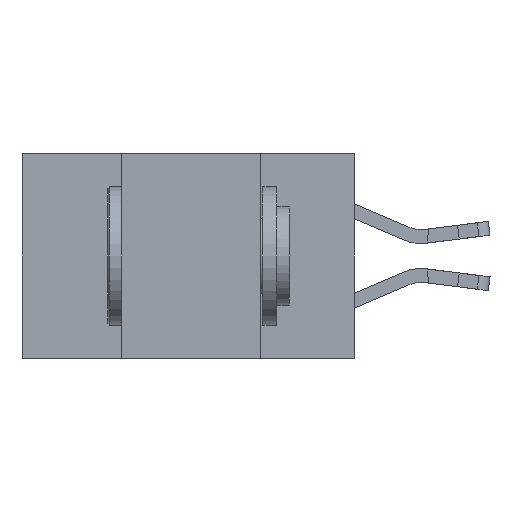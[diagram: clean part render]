
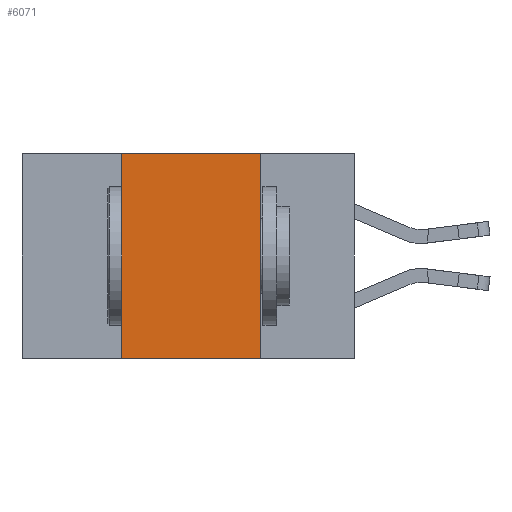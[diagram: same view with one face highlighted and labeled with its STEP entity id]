
A CAD part, left-side view. The second image highlights one B-rep face of the part: STEP entity #6071.
In plain terms, the highlighted planar face has unit normal (-1, 0, 0).
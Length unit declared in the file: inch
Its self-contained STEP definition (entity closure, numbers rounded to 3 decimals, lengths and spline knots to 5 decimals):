
#549 = DIRECTION ( 'NONE',  ( 0., -1., 0. ) ) ;
#946 = CARTESIAN_POINT ( 'NONE',  ( 0., 0.6, 0. ) ) ;
#1164 = CARTESIAN_POINT ( 'NONE',  ( 0., 0.17, 0. ) ) ;
#1494 = AXIS2_PLACEMENT_3D ( 'NONE', #2939, #2865, #2854 ) ;
#1776 = EDGE_CURVE ( 'NONE', #9136, #8596, #9429, .T. ) ;
#1821 = LINE ( 'NONE', #5766, #6699 ) ;
#2854 = DIRECTION ( 'NONE',  ( 0., 0., -1. ) ) ;
#2865 = DIRECTION ( 'NONE',  ( 1., 0., 0. ) ) ;
#2939 = CARTESIAN_POINT ( 'NONE',  ( 0., 0.6, 0. ) ) ;
#2973 = PLANE ( 'NONE',  #1494 ) ;
#3328 = FACE_OUTER_BOUND ( 'NONE', #4471, .T. ) ;
#3391 = VERTEX_POINT ( 'NONE', #1164 ) ;
#3568 = CARTESIAN_POINT ( 'NONE',  ( 0., 0.42, 0. ) ) ;
#3905 = VECTOR ( 'NONE', #13794, 39.37008 ) ;
#4190 = VERTEX_POINT ( 'NONE', #3568 ) ;
#4278 = EDGE_CURVE ( 'NONE', #4190, #3391, #4328, .T. ) ;
#4328 = LINE ( 'NONE', #946, #13691 ) ;
#4471 = EDGE_LOOP ( 'NONE', ( #10230, #9326, #13396, #7940 ) ) ;
#5720 = DIRECTION ( 'NONE',  ( 0., 0., 1. ) ) ;
#5766 = CARTESIAN_POINT ( 'NONE',  ( 0., 0.42, -0.37 ) ) ;
#5889 = CARTESIAN_POINT ( 'NONE',  ( 0., 0.17, -0.37 ) ) ;
#6071 = ADVANCED_FACE ( 'NONE', ( #3328 ), #2973, .F. ) ;
#6699 = VECTOR ( 'NONE', #5720, 39.37008 ) ;
#7940 = ORIENTED_EDGE ( 'NONE', *, *, #1776, .T. ) ;
#8221 = CARTESIAN_POINT ( 'NONE',  ( 0., 0.42, -0.37 ) ) ;
#8596 = VERTEX_POINT ( 'NONE', #5889 ) ;
#9136 = VERTEX_POINT ( 'NONE', #8221 ) ;
#9326 = ORIENTED_EDGE ( 'NONE', *, *, #4278, .F. ) ;
#9429 = LINE ( 'NONE', #12671, #3905 ) ;
#10230 = ORIENTED_EDGE ( 'NONE', *, *, #13237, .F. ) ;
#11898 = VECTOR ( 'NONE', #12663, 39.37008 ) ;
#12663 = DIRECTION ( 'NONE',  ( 0., 0., -1. ) ) ;
#12671 = CARTESIAN_POINT ( 'NONE',  ( 0., 0.6, -0.37 ) ) ;
#12776 = CARTESIAN_POINT ( 'NONE',  ( 0., 0.17, -0.37 ) ) ;
#13237 = EDGE_CURVE ( 'NONE', #3391, #8596, #14882, .T. ) ;
#13396 = ORIENTED_EDGE ( 'NONE', *, *, #13979, .F. ) ;
#13691 = VECTOR ( 'NONE', #549, 39.37008 ) ;
#13794 = DIRECTION ( 'NONE',  ( 0., -1., 0. ) ) ;
#13979 = EDGE_CURVE ( 'NONE', #9136, #4190, #1821, .T. ) ;
#14882 = LINE ( 'NONE', #12776, #11898 ) ;
